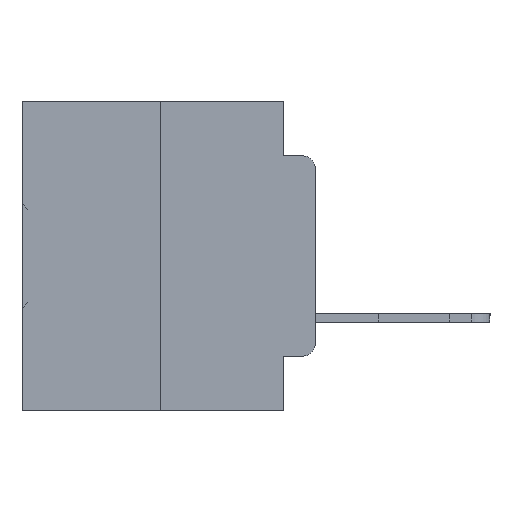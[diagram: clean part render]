
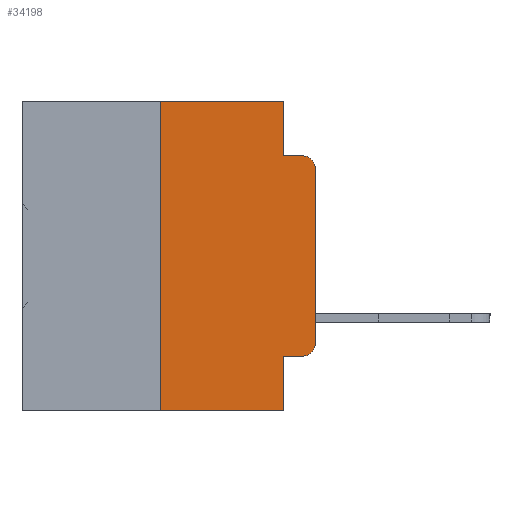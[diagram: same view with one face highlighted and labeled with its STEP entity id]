
A CAD part, left-side view. The second image highlights one B-rep face of the part: STEP entity #34198.
In plain terms, the highlighted planar face has unit normal (-1, 0, 0).
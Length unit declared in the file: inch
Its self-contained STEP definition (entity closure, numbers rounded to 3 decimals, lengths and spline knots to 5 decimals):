
#239 = DIRECTION ( 'NONE',  ( 0., -1., 0. ) ) ;
#271 = CARTESIAN_POINT ( 'NONE',  ( 0., 0.02, -0.4115 ) ) ;
#319 = ORIENTED_EDGE ( 'NONE', *, *, #4269, .T. ) ;
#491 = DIRECTION ( 'NONE',  ( 1., 0., 0. ) ) ;
#642 = DIRECTION ( 'NONE',  ( 0., 0., -1. ) ) ;
#904 = VERTEX_POINT ( 'NONE', #27994 ) ;
#1884 = CARTESIAN_POINT ( 'NONE',  ( 0., 0.473, -0.5 ) ) ;
#2559 = VERTEX_POINT ( 'NONE', #9799 ) ;
#2726 = CARTESIAN_POINT ( 'NONE',  ( 0., 0.473, 0. ) ) ;
#2924 = EDGE_CURVE ( 'NONE', #20814, #18499, #28364, .T. ) ;
#3046 = CIRCLE ( 'NONE', #14443, 0.02 ) ;
#4269 = EDGE_CURVE ( 'NONE', #36867, #28941, #30373, .T. ) ;
#5499 = EDGE_CURVE ( 'NONE', #12587, #13040, #16314, .T. ) ;
#5618 = EDGE_CURVE ( 'NONE', #13040, #36338, #3046, .T. ) ;
#5806 = EDGE_CURVE ( 'NONE', #904, #36338, #9277, .T. ) ;
#5876 = EDGE_CURVE ( 'NONE', #18499, #904, #27904, .T. ) ;
#5937 = EDGE_CURVE ( 'NONE', #36867, #20814, #25337, .T. ) ;
#5997 = EDGE_CURVE ( 'NONE', #2559, #28941, #16212, .T. ) ;
#6003 = EDGE_CURVE ( 'NONE', #2559, #33502, #21856, .T. ) ;
#6009 = EDGE_CURVE ( 'NONE', #33502, #12587, #14510, .T. ) ;
#6385 = ORIENTED_EDGE ( 'NONE', *, *, #5618, .T. ) ;
#6906 = VECTOR ( 'NONE', #239, 39.37008 ) ;
#7306 = CARTESIAN_POINT ( 'NONE',  ( 0., 0.02, -0.1085 ) ) ;
#7826 = VECTOR ( 'NONE', #26351, 39.37008 ) ;
#8904 = VECTOR ( 'NONE', #11754, 39.37008 ) ;
#9197 = VECTOR ( 'NONE', #33050, 39.37008 ) ;
#9277 = LINE ( 'NONE', #28034, #17574 ) ;
#9799 = CARTESIAN_POINT ( 'NONE',  ( 0., 0.051, -0.4115 ) ) ;
#9969 = CARTESIAN_POINT ( 'NONE',  ( 0., 0.473, 0. ) ) ;
#10269 = DIRECTION ( 'NONE',  ( 0., 0., -1. ) ) ;
#11470 = DIRECTION ( 'NONE',  ( 0., -1., 0. ) ) ;
#11754 = DIRECTION ( 'NONE',  ( 0., 0., 1. ) ) ;
#12558 = CARTESIAN_POINT ( 'NONE',  ( 0., 0.051, 0. ) ) ;
#12587 = VERTEX_POINT ( 'NONE', #19133 ) ;
#13040 = VERTEX_POINT ( 'NONE', #28869 ) ;
#13186 = VECTOR ( 'NONE', #31118, 39.37008 ) ;
#13313 = AXIS2_PLACEMENT_3D ( 'NONE', #9969, #491, #642 ) ;
#14443 = AXIS2_PLACEMENT_3D ( 'NONE', #7306, #26861, #10269 ) ;
#14510 = CIRCLE ( 'NONE', #20503, 0.02 ) ;
#14995 = CARTESIAN_POINT ( 'NONE',  ( 0., 0.25, 0. ) ) ;
#15459 = DIRECTION ( 'NONE',  ( -1., 0., 0. ) ) ;
#15759 = ORIENTED_EDGE ( 'NONE', *, *, #5806, .F. ) ;
#16199 = ORIENTED_EDGE ( 'NONE', *, *, #5997, .F. ) ;
#16212 = LINE ( 'NONE', #12558, #7826 ) ;
#16314 = LINE ( 'NONE', #28321, #8904 ) ;
#17517 = ORIENTED_EDGE ( 'NONE', *, *, #5876, .F. ) ;
#17574 = VECTOR ( 'NONE', #11470, 39.37008 ) ;
#18499 = VERTEX_POINT ( 'NONE', #24361 ) ;
#18916 = CARTESIAN_POINT ( 'NONE',  ( 0., 0.051, -0.5 ) ) ;
#19133 = CARTESIAN_POINT ( 'NONE',  ( 0., 0., -0.3915 ) ) ;
#19263 = ORIENTED_EDGE ( 'NONE', *, *, #2924, .F. ) ;
#19926 = EDGE_LOOP ( 'NONE', ( #27851, #6385, #15759, #17517, #19263, #35556, #319, #16199, #25322, #32549 ) ) ;
#20102 = DIRECTION ( 'NONE',  ( 0., -1., 0. ) ) ;
#20503 = AXIS2_PLACEMENT_3D ( 'NONE', #31947, #15459, #34707 ) ;
#20814 = VERTEX_POINT ( 'NONE', #31636 ) ;
#21856 = LINE ( 'NONE', #34586, #6906 ) ;
#22670 = CARTESIAN_POINT ( 'NONE',  ( 0., 0.02, -0.0885 ) ) ;
#24361 = CARTESIAN_POINT ( 'NONE',  ( 0., 0.051, 0. ) ) ;
#25322 = ORIENTED_EDGE ( 'NONE', *, *, #6003, .T. ) ;
#25337 = LINE ( 'NONE', #14995, #33442 ) ;
#26351 = DIRECTION ( 'NONE',  ( 0., 0., -1. ) ) ;
#26861 = DIRECTION ( 'NONE',  ( -1., 0., 0. ) ) ;
#27851 = ORIENTED_EDGE ( 'NONE', *, *, #5499, .T. ) ;
#27904 = LINE ( 'NONE', #30993, #13186 ) ;
#27994 = CARTESIAN_POINT ( 'NONE',  ( 0., 0.051, -0.0885 ) ) ;
#28034 = CARTESIAN_POINT ( 'NONE',  ( 0., 0.051, -0.0885 ) ) ;
#28321 = CARTESIAN_POINT ( 'NONE',  ( 0., 0., 0. ) ) ;
#28364 = LINE ( 'NONE', #2726, #34758 ) ;
#28869 = CARTESIAN_POINT ( 'NONE',  ( 0., 0., -0.1085 ) ) ;
#28924 = FACE_OUTER_BOUND ( 'NONE', #19926, .T. ) ;
#28941 = VERTEX_POINT ( 'NONE', #18916 ) ;
#30373 = LINE ( 'NONE', #1884, #9197 ) ;
#30993 = CARTESIAN_POINT ( 'NONE',  ( 0., 0.051, 0. ) ) ;
#31118 = DIRECTION ( 'NONE',  ( 0., 0., -1. ) ) ;
#31476 = DIRECTION ( 'NONE',  ( 0., 0., 1. ) ) ;
#31636 = CARTESIAN_POINT ( 'NONE',  ( 0., 0.25, 0. ) ) ;
#31947 = CARTESIAN_POINT ( 'NONE',  ( 0., 0.02, -0.3915 ) ) ;
#32028 = PLANE ( 'NONE',  #13313 ) ;
#32549 = ORIENTED_EDGE ( 'NONE', *, *, #6009, .T. ) ;
#33050 = DIRECTION ( 'NONE',  ( 0., -1., 0. ) ) ;
#33442 = VECTOR ( 'NONE', #31476, 39.37008 ) ;
#33502 = VERTEX_POINT ( 'NONE', #271 ) ;
#34198 = ADVANCED_FACE ( 'NONE', ( #28924 ), #32028, .F. ) ;
#34586 = CARTESIAN_POINT ( 'NONE',  ( 0., 0.051, -0.4115 ) ) ;
#34707 = DIRECTION ( 'NONE',  ( 0., 0., -1. ) ) ;
#34758 = VECTOR ( 'NONE', #20102, 39.37008 ) ;
#35556 = ORIENTED_EDGE ( 'NONE', *, *, #5937, .F. ) ;
#35568 = CARTESIAN_POINT ( 'NONE',  ( 0., 0.25, -0.5 ) ) ;
#36338 = VERTEX_POINT ( 'NONE', #22670 ) ;
#36867 = VERTEX_POINT ( 'NONE', #35568 ) ;
